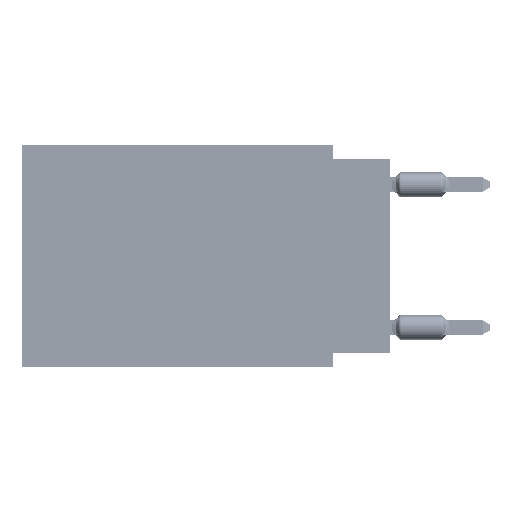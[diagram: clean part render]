
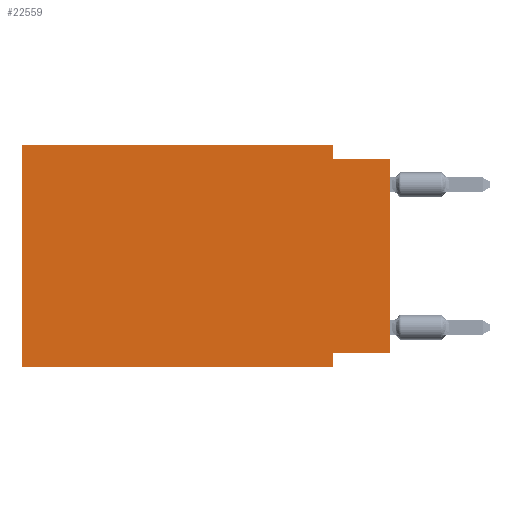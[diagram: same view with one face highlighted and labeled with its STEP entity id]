
A CAD part, left-side view. The second image highlights one B-rep face of the part: STEP entity #22559.
In plain terms, the highlighted planar face has unit normal (-1, 0, 0).
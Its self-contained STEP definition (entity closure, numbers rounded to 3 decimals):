
#504 = DIRECTION ( 'NONE',  ( 0., 0., -1. ) ) ;
#3682 = EDGE_CURVE ( 'NONE', #25408, #26537, #53419, .T. ) ;
#5995 = LINE ( 'NONE', #7004, #44108 ) ;
#6269 = LINE ( 'NONE', #38720, #30667 ) ;
#6664 = LINE ( 'NONE', #54830, #38167 ) ;
#7004 = CARTESIAN_POINT ( 'NONE',  ( 0., 16.383, 0. ) ) ;
#10613 = EDGE_CURVE ( 'NONE', #19607, #54789, #42476, .T. ) ;
#11540 = EDGE_CURVE ( 'NONE', #38251, #31114, #6664, .T. ) ;
#14226 = EDGE_CURVE ( 'NONE', #19607, #18756, #5995, .T. ) ;
#15922 = DIRECTION ( 'NONE',  ( 0., -1., 0. ) ) ;
#16152 = CARTESIAN_POINT ( 'NONE',  ( 0., 0., -9.271 ) ) ;
#17138 = DIRECTION ( 'NONE',  ( 0., 1., 0. ) ) ;
#17318 = CARTESIAN_POINT ( 'NONE',  ( 0., 2.54, 0. ) ) ;
#17594 = EDGE_CURVE ( 'NONE', #38251, #26537, #34175, .T. ) ;
#17893 = CARTESIAN_POINT ( 'NONE',  ( 0., 2.54, 0. ) ) ;
#18756 = VERTEX_POINT ( 'NONE', #58756 ) ;
#19607 = VERTEX_POINT ( 'NONE', #33672 ) ;
#20134 = ORIENTED_EDGE ( 'NONE', *, *, #17594, .T. ) ;
#21307 = ORIENTED_EDGE ( 'NONE', *, *, #32197, .F. ) ;
#22075 = DIRECTION ( 'NONE',  ( 0., -1., 0. ) ) ;
#22489 = DIRECTION ( 'NONE',  ( 1., 0., 0. ) ) ;
#22559 = ADVANCED_FACE ( 'NONE', ( #43443 ), #49707, .F. ) ;
#22801 = VECTOR ( 'NONE', #32697, 1000. ) ;
#23052 = ORIENTED_EDGE ( 'NONE', *, *, #10613, .T. ) ;
#25408 = VERTEX_POINT ( 'NONE', #58669 ) ;
#26537 = VERTEX_POINT ( 'NONE', #67455 ) ;
#26541 = CARTESIAN_POINT ( 'NONE',  ( 0., 0., -0.635 ) ) ;
#27132 = CARTESIAN_POINT ( 'NONE',  ( 0., 2.54, -9.271 ) ) ;
#27310 = CARTESIAN_POINT ( 'NONE',  ( 0., 16.383, 0. ) ) ;
#27566 = DIRECTION ( 'NONE',  ( 0., 0., 1. ) ) ;
#28713 = EDGE_CURVE ( 'NONE', #59567, #25408, #39301, .T. ) ;
#28856 = ORIENTED_EDGE ( 'NONE', *, *, #14226, .F. ) ;
#30667 = VECTOR ( 'NONE', #42937, 1000. ) ;
#31114 = VERTEX_POINT ( 'NONE', #27132 ) ;
#32197 = EDGE_CURVE ( 'NONE', #18756, #59567, #48613, .T. ) ;
#32697 = DIRECTION ( 'NONE',  ( 0., 0., -1. ) ) ;
#33672 = CARTESIAN_POINT ( 'NONE',  ( 0., 16.383, -9.906 ) ) ;
#34175 = LINE ( 'NONE', #50250, #49824 ) ;
#38167 = VECTOR ( 'NONE', #17138, 1000. ) ;
#38251 = VERTEX_POINT ( 'NONE', #16152 ) ;
#38720 = CARTESIAN_POINT ( 'NONE',  ( 0., 2.54, -9.906 ) ) ;
#39301 = LINE ( 'NONE', #17318, #22801 ) ;
#42476 = LINE ( 'NONE', #52939, #54676 ) ;
#42937 = DIRECTION ( 'NONE',  ( 0., 0., -1. ) ) ;
#43443 = FACE_OUTER_BOUND ( 'NONE', #46959, .T. ) ;
#44108 = VECTOR ( 'NONE', #59397, 1000. ) ;
#45290 = VECTOR ( 'NONE', #68802, 1000. ) ;
#46607 = CARTESIAN_POINT ( 'NONE',  ( 0., 2.54, -9.906 ) ) ;
#46959 = EDGE_LOOP ( 'NONE', ( #20134, #63639, #68295, #21307, #28856, #23052, #66154, #62200 ) ) ;
#48337 = CARTESIAN_POINT ( 'NONE',  ( 0., 16.383, 0. ) ) ;
#48613 = LINE ( 'NONE', #27310, #57664 ) ;
#49707 = PLANE ( 'NONE',  #59228 ) ;
#49824 = VECTOR ( 'NONE', #27566, 1000. ) ;
#50250 = CARTESIAN_POINT ( 'NONE',  ( 0., 0., 0. ) ) ;
#51441 = EDGE_CURVE ( 'NONE', #31114, #54789, #6269, .T. ) ;
#52939 = CARTESIAN_POINT ( 'NONE',  ( 0., 16.383, -9.906 ) ) ;
#53419 = LINE ( 'NONE', #26541, #45290 ) ;
#54676 = VECTOR ( 'NONE', #15922, 1000. ) ;
#54789 = VERTEX_POINT ( 'NONE', #46607 ) ;
#54830 = CARTESIAN_POINT ( 'NONE',  ( 0., 0., -9.271 ) ) ;
#57664 = VECTOR ( 'NONE', #22075, 1000. ) ;
#58669 = CARTESIAN_POINT ( 'NONE',  ( 0., 2.54, -0.635 ) ) ;
#58756 = CARTESIAN_POINT ( 'NONE',  ( 0., 16.383, 0. ) ) ;
#59228 = AXIS2_PLACEMENT_3D ( 'NONE', #48337, #22489, #504 ) ;
#59397 = DIRECTION ( 'NONE',  ( 0., 0., 1. ) ) ;
#59567 = VERTEX_POINT ( 'NONE', #17893 ) ;
#62200 = ORIENTED_EDGE ( 'NONE', *, *, #11540, .F. ) ;
#63639 = ORIENTED_EDGE ( 'NONE', *, *, #3682, .F. ) ;
#66154 = ORIENTED_EDGE ( 'NONE', *, *, #51441, .F. ) ;
#67455 = CARTESIAN_POINT ( 'NONE',  ( 0., 0., -0.635 ) ) ;
#68295 = ORIENTED_EDGE ( 'NONE', *, *, #28713, .F. ) ;
#68802 = DIRECTION ( 'NONE',  ( 0., -1., 0. ) ) ;
